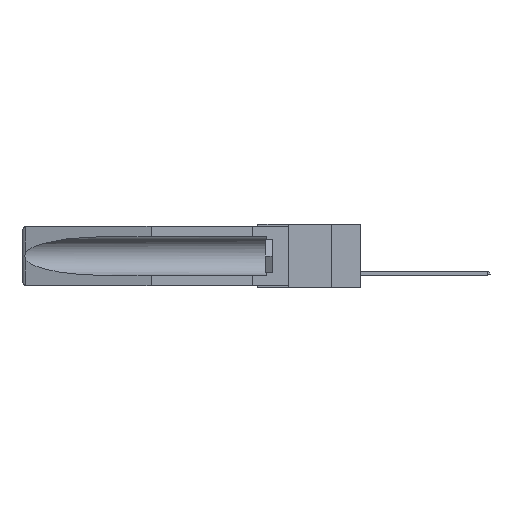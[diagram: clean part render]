
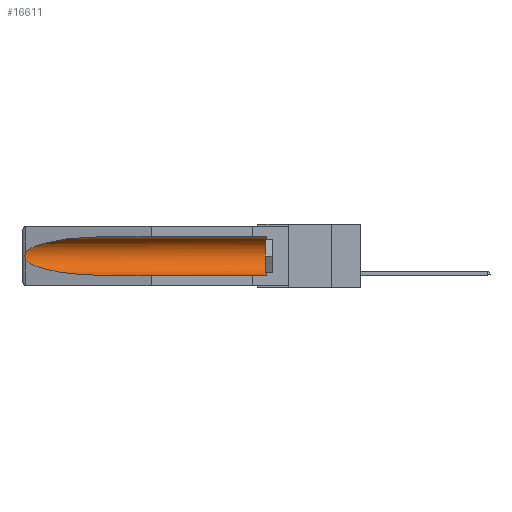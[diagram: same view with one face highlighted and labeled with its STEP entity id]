
A CAD part, left-side view. The second image highlights one B-rep face of the part: STEP entity #16611.
In plain terms, the highlighted cylindrical face has radius 2.857 mm (diameter 5.715 mm), a partial arc.
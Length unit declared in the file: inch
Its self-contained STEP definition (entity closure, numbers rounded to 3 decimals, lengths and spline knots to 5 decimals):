
#193 =( BOUNDED_CURVE ( )  B_SPLINE_CURVE ( 3, ( #4616, #8472, #12251, #12568 ),
 .UNSPECIFIED., .F., .F. ) 
 B_SPLINE_CURVE_WITH_KNOTS ( ( 4, 4 ),
 ( 0.1948, 1.5708 ),
 .UNSPECIFIED. ) 
 CURVE ( )  GEOMETRIC_REPRESENTATION_ITEM ( )  RATIONAL_B_SPLINE_CURVE ( ( 1., 0.848, 0.848, 1. ) ) 
 REPRESENTATION_ITEM ( '' )  );
#511 = CARTESIAN_POINT ( 'NONE',  ( 0.155, 1.07973, -0.059 ) ) ;
#660 = B_SPLINE_CURVE_WITH_KNOTS ( 'NONE', 3,
 ( #23326, #9759, #13882, #23485, #10007, #6023, #15587, #5931, #4053, #15755 ),
 .UNSPECIFIED., .F., .F.,
 ( 4, 2, 2, 2, 4 ),
 ( 0., 0.00029, 0.00058, 0.00087, 0.00117 ),
 .UNSPECIFIED. ) ;
#1365 = EDGE_CURVE ( 'NONE', #23380, #2424, #193, .T. ) ;
#1420 =( BOUNDED_CURVE ( )  B_SPLINE_CURVE ( 3, ( #511, #6274, #16082, #4470 ),
 .UNSPECIFIED., .F., .F. ) 
 B_SPLINE_CURVE_WITH_KNOTS ( ( 4, 4 ),
 ( 4.71239, 6.08839 ),
 .UNSPECIFIED. ) 
 CURVE ( )  GEOMETRIC_REPRESENTATION_ITEM ( )  RATIONAL_B_SPLINE_CURVE ( ( 1., 0.848, 0.848, 1. ) ) 
 REPRESENTATION_ITEM ( '' )  );
#1642 = DIRECTION ( 'NONE',  ( 0., 1., 0. ) ) ;
#2209 = ORIENTED_EDGE ( 'NONE', *, *, #16233, .T. ) ;
#2424 = VERTEX_POINT ( 'NONE', #14045 ) ;
#2611 = CARTESIAN_POINT ( 'NONE',  ( 0.155, 1.07973, -0.059 ) ) ;
#2767 = DIRECTION ( 'NONE',  ( 0., 1., 0. ) ) ;
#3138 = LINE ( 'NONE', #19918, #18859 ) ;
#3442 = LINE ( 'NONE', #24785, #14952 ) ;
#4053 = CARTESIAN_POINT ( 'NONE',  ( 0.26597, 1.5296, -0.19026 ) ) ;
#4076 = CARTESIAN_POINT ( 'NONE',  ( 0.155, 0.126, -0.1715 ) ) ;
#4470 = CARTESIAN_POINT ( 'NONE',  ( 0.26537, 1.52718, -0.14972 ) ) ;
#4616 = CARTESIAN_POINT ( 'NONE',  ( 0.26537, 1.52718, -0.19328 ) ) ;
#4754 = VERTEX_POINT ( 'NONE', #17613 ) ;
#5109 = EDGE_CURVE ( 'NONE', #13139, #23380, #660, .T. ) ;
#5297 = VERTEX_POINT ( 'NONE', #2611 ) ;
#5931 = CARTESIAN_POINT ( 'NONE',  ( 0.26655, 1.53094, -0.18657 ) ) ;
#6023 = CARTESIAN_POINT ( 'NONE',  ( 0.2675, 1.53308, -0.17534 ) ) ;
#6274 = CARTESIAN_POINT ( 'NONE',  ( 0.21114, 1.30732, -0.059 ) ) ;
#8138 = DIRECTION ( 'NONE',  ( 0., 0., 1. ) ) ;
#8472 = CARTESIAN_POINT ( 'NONE',  ( 0.25451, 1.48313, -0.24835 ) ) ;
#8509 = CARTESIAN_POINT ( 'NONE',  ( 0.26537, 1.52718, -0.14972 ) ) ;
#9178 = CYLINDRICAL_SURFACE ( 'NONE', #17861, 0.1125 ) ;
#9759 = CARTESIAN_POINT ( 'NONE',  ( 0.26597, 1.52961, -0.15275 ) ) ;
#10007 = CARTESIAN_POINT ( 'NONE',  ( 0.2675, 1.53308, -0.16763 ) ) ;
#10983 = EDGE_CURVE ( 'NONE', #5297, #13139, #1420, .T. ) ;
#11769 = CARTESIAN_POINT ( 'NONE',  ( 0.26537, 1.52718, -0.19328 ) ) ;
#11915 = DIRECTION ( 'NONE',  ( 0., 1., 0. ) ) ;
#12251 = CARTESIAN_POINT ( 'NONE',  ( 0.21114, 1.30732, -0.284 ) ) ;
#12568 = CARTESIAN_POINT ( 'NONE',  ( 0.155, 1.07973, -0.284 ) ) ;
#13139 = VERTEX_POINT ( 'NONE', #8509 ) ;
#13725 = FACE_OUTER_BOUND ( 'NONE', #18239, .T. ) ;
#13815 = DIRECTION ( 'NONE',  ( 0., 0., 1. ) ) ;
#13882 = CARTESIAN_POINT ( 'NONE',  ( 0.26654, 1.53092, -0.15636 ) ) ;
#14045 = CARTESIAN_POINT ( 'NONE',  ( 0.155, 1.07973, -0.284 ) ) ;
#14952 = VECTOR ( 'NONE', #1642, 39.37008 ) ;
#15351 = AXIS2_PLACEMENT_3D ( 'NONE', #4076, #17779, #13815 ) ;
#15587 = CARTESIAN_POINT ( 'NONE',  ( 0.2673, 1.53269, -0.17917 ) ) ;
#15755 = CARTESIAN_POINT ( 'NONE',  ( 0.26537, 1.52718, -0.19328 ) ) ;
#15801 = ORIENTED_EDGE ( 'NONE', *, *, #21981, .T. ) ;
#16053 = ORIENTED_EDGE ( 'NONE', *, *, #10983, .T. ) ;
#16058 = EDGE_CURVE ( 'NONE', #18102, #2424, #3138, .T. ) ;
#16082 = CARTESIAN_POINT ( 'NONE',  ( 0.25451, 1.48313, -0.09465 ) ) ;
#16233 = EDGE_CURVE ( 'NONE', #4754, #5297, #3442, .T. ) ;
#16611 = ADVANCED_FACE ( 'NONE', ( #13725 ), #9178, .F. ) ;
#16827 = ORIENTED_EDGE ( 'NONE', *, *, #1365, .T. ) ;
#17613 = CARTESIAN_POINT ( 'NONE',  ( 0.155, 0.126, -0.059 ) ) ;
#17779 = DIRECTION ( 'NONE',  ( 0., -1., 0. ) ) ;
#17861 = AXIS2_PLACEMENT_3D ( 'NONE', #21514, #11915, #8138 ) ;
#18102 = VERTEX_POINT ( 'NONE', #19949 ) ;
#18239 = EDGE_LOOP ( 'NONE', ( #16053, #19695, #16827, #18664, #15801, #2209 ) ) ;
#18664 = ORIENTED_EDGE ( 'NONE', *, *, #16058, .F. ) ;
#18859 = VECTOR ( 'NONE', #2767, 39.37008 ) ;
#19460 = CIRCLE ( 'NONE', #15351, 0.1125 ) ;
#19695 = ORIENTED_EDGE ( 'NONE', *, *, #5109, .T. ) ;
#19918 = CARTESIAN_POINT ( 'NONE',  ( 0.155, -0.30754, -0.284 ) ) ;
#19949 = CARTESIAN_POINT ( 'NONE',  ( 0.155, 0.126, -0.284 ) ) ;
#21514 = CARTESIAN_POINT ( 'NONE',  ( 0.155, -0.30754, -0.1715 ) ) ;
#21981 = EDGE_CURVE ( 'NONE', #18102, #4754, #19460, .T. ) ;
#23326 = CARTESIAN_POINT ( 'NONE',  ( 0.26537, 1.52718, -0.14972 ) ) ;
#23380 = VERTEX_POINT ( 'NONE', #11769 ) ;
#23485 = CARTESIAN_POINT ( 'NONE',  ( 0.2673, 1.5327, -0.16383 ) ) ;
#24785 = CARTESIAN_POINT ( 'NONE',  ( 0.155, -0.30754, -0.059 ) ) ;
